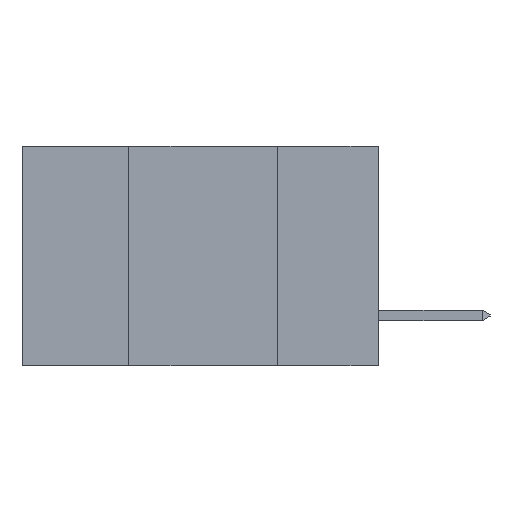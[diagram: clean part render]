
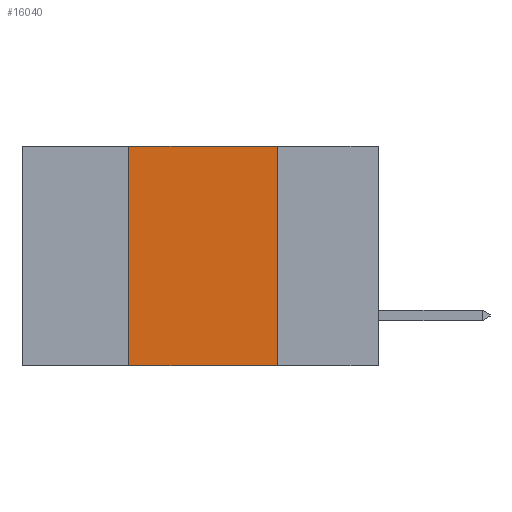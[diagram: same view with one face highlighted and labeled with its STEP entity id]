
A CAD part, left-side view. The second image highlights one B-rep face of the part: STEP entity #16040.
In plain terms, the highlighted planar face has unit normal (-1, 0, 0).
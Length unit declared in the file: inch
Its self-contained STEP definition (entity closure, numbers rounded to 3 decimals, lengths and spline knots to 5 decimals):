
#70 = VECTOR ( 'NONE', #17665, 39.37008 ) ;
#609 = LINE ( 'NONE', #3207, #70 ) ;
#1729 = PLANE ( 'NONE',  #4997 ) ;
#1741 = FACE_OUTER_BOUND ( 'NONE', #21923, .T. ) ;
#3125 = EDGE_CURVE ( 'NONE', #4530, #16508, #609, .T. ) ;
#3207 = CARTESIAN_POINT ( 'NONE',  ( 0., 0.42, 0. ) ) ;
#3238 = ORIENTED_EDGE ( 'NONE', *, *, #15317, .F. ) ;
#3488 = CARTESIAN_POINT ( 'NONE',  ( 0., 0.42, -0.37 ) ) ;
#4269 = EDGE_CURVE ( 'NONE', #6308, #11046, #8139, .T. ) ;
#4530 = VERTEX_POINT ( 'NONE', #3488 ) ;
#4585 = CARTESIAN_POINT ( 'NONE',  ( 0., 0.6, 0. ) ) ;
#4997 = AXIS2_PLACEMENT_3D ( 'NONE', #4585, #15558, #5197 ) ;
#5197 = DIRECTION ( 'NONE',  ( 0., 0., -1. ) ) ;
#5885 = DIRECTION ( 'NONE',  ( 0., -1., 0. ) ) ;
#6308 = VERTEX_POINT ( 'NONE', #9258 ) ;
#7250 = ORIENTED_EDGE ( 'NONE', *, *, #4269, .F. ) ;
#7626 = CARTESIAN_POINT ( 'NONE',  ( 0., 0.6, 0. ) ) ;
#8139 = LINE ( 'NONE', #15981, #16780 ) ;
#9258 = CARTESIAN_POINT ( 'NONE',  ( 0., 0.17, 0. ) ) ;
#11046 = VERTEX_POINT ( 'NONE', #19772 ) ;
#13003 = ORIENTED_EDGE ( 'NONE', *, *, #21944, .T. ) ;
#14511 = DIRECTION ( 'NONE',  ( 0., 0., -1. ) ) ;
#14807 = CARTESIAN_POINT ( 'NONE',  ( 0., 0.6, -0.37 ) ) ;
#15317 = EDGE_CURVE ( 'NONE', #16508, #6308, #17424, .T. ) ;
#15558 = DIRECTION ( 'NONE',  ( 1., 0., 0. ) ) ;
#15981 = CARTESIAN_POINT ( 'NONE',  ( 0., 0.17, 0. ) ) ;
#16040 = ADVANCED_FACE ( 'NONE', ( #1741 ), #1729, .F. ) ;
#16508 = VERTEX_POINT ( 'NONE', #18499 ) ;
#16517 = DIRECTION ( 'NONE',  ( 0., -1., 0. ) ) ;
#16780 = VECTOR ( 'NONE', #14511, 39.37008 ) ;
#17011 = ORIENTED_EDGE ( 'NONE', *, *, #3125, .F. ) ;
#17093 = VECTOR ( 'NONE', #16517, 39.37008 ) ;
#17424 = LINE ( 'NONE', #7626, #21379 ) ;
#17665 = DIRECTION ( 'NONE',  ( 0., 0., 1. ) ) ;
#18499 = CARTESIAN_POINT ( 'NONE',  ( 0., 0.42, 0. ) ) ;
#19772 = CARTESIAN_POINT ( 'NONE',  ( 0., 0.17, -0.37 ) ) ;
#21379 = VECTOR ( 'NONE', #5885, 39.37008 ) ;
#21582 = LINE ( 'NONE', #14807, #17093 ) ;
#21923 = EDGE_LOOP ( 'NONE', ( #7250, #3238, #17011, #13003 ) ) ;
#21944 = EDGE_CURVE ( 'NONE', #4530, #11046, #21582, .T. ) ;
